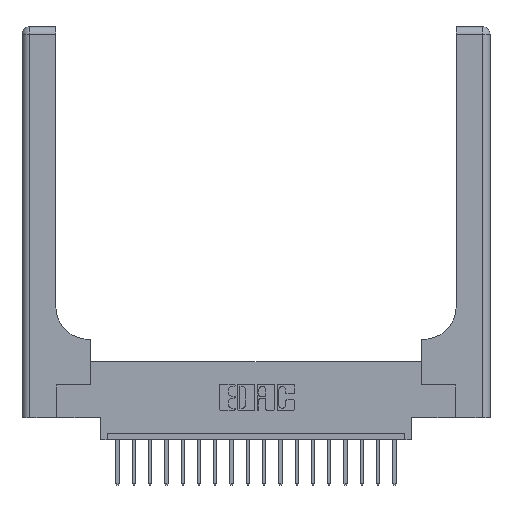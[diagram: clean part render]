
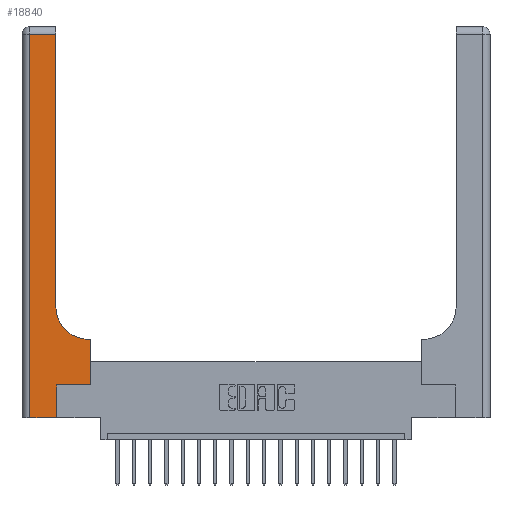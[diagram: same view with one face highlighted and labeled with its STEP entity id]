
A CAD part, top view. The second image highlights one B-rep face of the part: STEP entity #18840.
In plain terms, the highlighted planar face has unit normal (0, 0, 1).
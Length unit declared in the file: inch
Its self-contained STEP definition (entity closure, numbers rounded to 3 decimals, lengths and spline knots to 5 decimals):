
#405 = EDGE_CURVE ( 'NONE', #13825, #18093, #15588, .T. ) ;
#408 = LINE ( 'NONE', #16191, #1106 ) ;
#1025 = CARTESIAN_POINT ( 'NONE',  ( 0.26, 0.85, 0.37 ) ) ;
#1106 = VECTOR ( 'NONE', #9988, 39.37008 ) ;
#1145 = LINE ( 'NONE', #7533, #13819 ) ;
#1636 = CARTESIAN_POINT ( 'NONE',  ( 0., 3., 0.37 ) ) ;
#1811 = VERTEX_POINT ( 'NONE', #12427 ) ;
#1836 = ORIENTED_EDGE ( 'NONE', *, *, #15992, .T. ) ;
#1940 = FACE_OUTER_BOUND ( 'NONE', #8266, .T. ) ;
#1994 = LINE ( 'NONE', #12429, #6062 ) ;
#2540 = LINE ( 'NONE', #16309, #13535 ) ;
#2649 = VERTEX_POINT ( 'NONE', #12114 ) ;
#2709 = CARTESIAN_POINT ( 'NONE',  ( 0.26, 0.6, 0.37 ) ) ;
#2856 = CARTESIAN_POINT ( 'NONE',  ( 0.265, 0., 0.37 ) ) ;
#3149 = CARTESIAN_POINT ( 'NONE',  ( 0.26, 2.94, 0.37 ) ) ;
#3190 = DIRECTION ( 'NONE',  ( 0., 0., -1. ) ) ;
#3283 = VERTEX_POINT ( 'NONE', #2856 ) ;
#3634 = DIRECTION ( 'NONE',  ( 0., 0., -1. ) ) ;
#4657 = EDGE_CURVE ( 'NONE', #18093, #17000, #7586, .T. ) ;
#5180 = VERTEX_POINT ( 'NONE', #14259 ) ;
#6062 = VECTOR ( 'NONE', #15220, 39.37008 ) ;
#6348 = ORIENTED_EDGE ( 'NONE', *, *, #17417, .T. ) ;
#6553 = LINE ( 'NONE', #2709, #18005 ) ;
#6674 = AXIS2_PLACEMENT_3D ( 'NONE', #18619, #3634, #6697 ) ;
#6697 = DIRECTION ( 'NONE',  ( 1., 0., 0. ) ) ;
#6734 = CARTESIAN_POINT ( 'NONE',  ( 0.26, 3., 0.37 ) ) ;
#7064 = VERTEX_POINT ( 'NONE', #14926 ) ;
#7179 = DIRECTION ( 'NONE',  ( 1., 0., 0. ) ) ;
#7315 = ORIENTED_EDGE ( 'NONE', *, *, #10916, .T. ) ;
#7424 = CARTESIAN_POINT ( 'NONE',  ( 0.528, 0.25, 0.37 ) ) ;
#7533 = CARTESIAN_POINT ( 'NONE',  ( 0.265, 0., 0.37 ) ) ;
#7586 = LINE ( 'NONE', #6734, #10927 ) ;
#7597 = ORIENTED_EDGE ( 'NONE', *, *, #12032, .T. ) ;
#7970 = ORIENTED_EDGE ( 'NONE', *, *, #405, .T. ) ;
#8266 = EDGE_LOOP ( 'NONE', ( #13145, #9007, #1836, #7597, #10238, #13448, #7315, #6348, #7970 ) ) ;
#8427 = VECTOR ( 'NONE', #9095, 39.37008 ) ;
#8593 = DIRECTION ( 'NONE',  ( -1., 0., 0. ) ) ;
#8627 = LINE ( 'NONE', #14666, #18647 ) ;
#9007 = ORIENTED_EDGE ( 'NONE', *, *, #10659, .T. ) ;
#9095 = DIRECTION ( 'NONE',  ( 0., 1., 0. ) ) ;
#9988 = DIRECTION ( 'NONE',  ( 0., -1., 0. ) ) ;
#10238 = ORIENTED_EDGE ( 'NONE', *, *, #15359, .T. ) ;
#10659 = EDGE_CURVE ( 'NONE', #17000, #5180, #1994, .T. ) ;
#10916 = EDGE_CURVE ( 'NONE', #1811, #7064, #19398, .T. ) ;
#10927 = VECTOR ( 'NONE', #14346, 39.37008 ) ;
#11005 = DIRECTION ( 'NONE',  ( 0., 1., 0. ) ) ;
#12032 = EDGE_CURVE ( 'NONE', #16100, #3283, #8627, .T. ) ;
#12054 = CARTESIAN_POINT ( 'NONE',  ( 0.06, 0., 0.37 ) ) ;
#12114 = CARTESIAN_POINT ( 'NONE',  ( 0.265, 0.25, 0.37 ) ) ;
#12427 = CARTESIAN_POINT ( 'NONE',  ( 0.528, 0.25, 0.37 ) ) ;
#12429 = CARTESIAN_POINT ( 'NONE',  ( 0., 2.94, 0.37 ) ) ;
#13145 = ORIENTED_EDGE ( 'NONE', *, *, #4657, .T. ) ;
#13282 = CARTESIAN_POINT ( 'NONE',  ( 0.51, 0.6, 0.37 ) ) ;
#13448 = ORIENTED_EDGE ( 'NONE', *, *, #16056, .T. ) ;
#13535 = VECTOR ( 'NONE', #7179, 39.37008 ) ;
#13819 = VECTOR ( 'NONE', #11005, 39.37008 ) ;
#13825 = VERTEX_POINT ( 'NONE', #13282 ) ;
#13869 = DIRECTION ( 'NONE',  ( -1., 0., 0. ) ) ;
#14259 = CARTESIAN_POINT ( 'NONE',  ( 0.06, 2.94, 0.37 ) ) ;
#14346 = DIRECTION ( 'NONE',  ( 0., 1., 0. ) ) ;
#14666 = CARTESIAN_POINT ( 'NONE',  ( 0., 0., 0.37 ) ) ;
#14926 = CARTESIAN_POINT ( 'NONE',  ( 0.528, 0.6, 0.37 ) ) ;
#15220 = DIRECTION ( 'NONE',  ( -1., 0., 0. ) ) ;
#15359 = EDGE_CURVE ( 'NONE', #3283, #2649, #1145, .T. ) ;
#15588 = CIRCLE ( 'NONE', #6674, 0.25 ) ;
#15992 = EDGE_CURVE ( 'NONE', #5180, #16100, #408, .T. ) ;
#16056 = EDGE_CURVE ( 'NONE', #2649, #1811, #2540, .T. ) ;
#16100 = VERTEX_POINT ( 'NONE', #12054 ) ;
#16191 = CARTESIAN_POINT ( 'NONE',  ( 0.06, 3., 0.37 ) ) ;
#16309 = CARTESIAN_POINT ( 'NONE',  ( 0.265, 0.25, 0.37 ) ) ;
#16786 = PLANE ( 'NONE',  #18490 ) ;
#17000 = VERTEX_POINT ( 'NONE', #3149 ) ;
#17417 = EDGE_CURVE ( 'NONE', #7064, #13825, #6553, .T. ) ;
#18005 = VECTOR ( 'NONE', #8593, 39.37008 ) ;
#18093 = VERTEX_POINT ( 'NONE', #1025 ) ;
#18490 = AXIS2_PLACEMENT_3D ( 'NONE', #1636, #3190, #13869 ) ;
#18619 = CARTESIAN_POINT ( 'NONE',  ( 0.51, 0.85, 0.37 ) ) ;
#18647 = VECTOR ( 'NONE', #19500, 39.37008 ) ;
#18840 = ADVANCED_FACE ( 'NONE', ( #1940 ), #16786, .F. ) ;
#19398 = LINE ( 'NONE', #7424, #8427 ) ;
#19500 = DIRECTION ( 'NONE',  ( 1., 0., 0. ) ) ;
